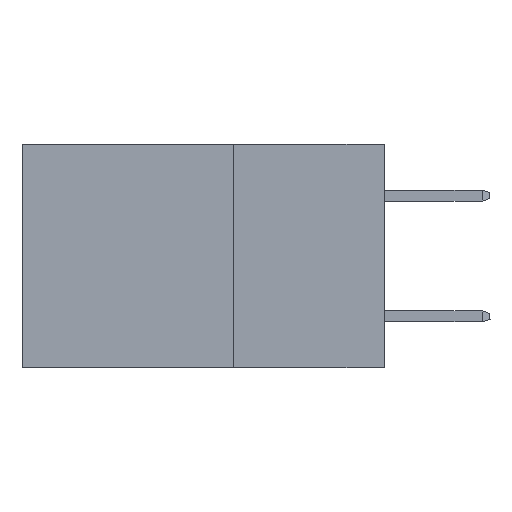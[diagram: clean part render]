
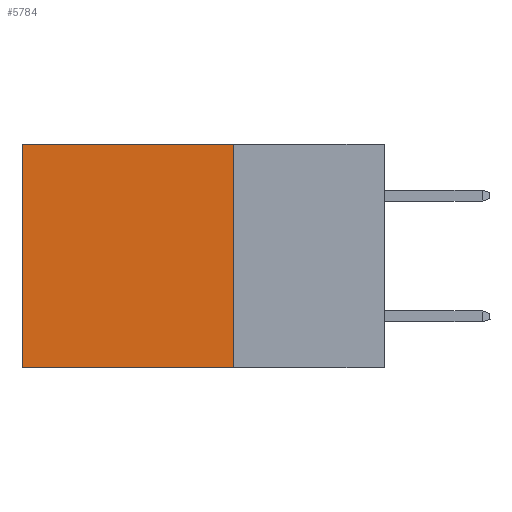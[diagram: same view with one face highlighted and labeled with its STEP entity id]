
A CAD part, left-side view. The second image highlights one B-rep face of the part: STEP entity #5784.
In plain terms, the highlighted planar face has unit normal (-1, 0, 0).
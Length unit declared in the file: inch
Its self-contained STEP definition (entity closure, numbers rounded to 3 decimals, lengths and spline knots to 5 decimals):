
#295 = PLANE ( 'NONE',  #4441 ) ;
#1437 = ORIENTED_EDGE ( 'NONE', *, *, #13617, .T. ) ;
#2033 = CARTESIAN_POINT ( 'NONE',  ( 0.2615, 0.25, -0.37 ) ) ;
#2458 = CARTESIAN_POINT ( 'NONE',  ( 0.2615, 0.25, 0. ) ) ;
#2679 = DIRECTION ( 'NONE',  ( 0., 0., -1. ) ) ;
#3398 = DIRECTION ( 'NONE',  ( 0., 1., 0. ) ) ;
#3536 = VECTOR ( 'NONE', #3398, 39.37008 ) ;
#3764 = DIRECTION ( 'NONE',  ( 1., 0., 0. ) ) ;
#4081 = LINE ( 'NONE', #8457, #3536 ) ;
#4148 = VERTEX_POINT ( 'NONE', #19362 ) ;
#4441 = AXIS2_PLACEMENT_3D ( 'NONE', #2033, #3764, #15387 ) ;
#5784 = ADVANCED_FACE ( 'NONE', ( #16815 ), #295, .F. ) ;
#7054 = EDGE_CURVE ( 'NONE', #9279, #13821, #4081, .T. ) ;
#7188 = VERTEX_POINT ( 'NONE', #13711 ) ;
#7354 = CARTESIAN_POINT ( 'NONE',  ( 0.2615, 0.25, -0.37 ) ) ;
#7905 = ORIENTED_EDGE ( 'NONE', *, *, #19389, .F. ) ;
#8277 = LINE ( 'NONE', #7354, #12148 ) ;
#8408 = LINE ( 'NONE', #19126, #16586 ) ;
#8457 = CARTESIAN_POINT ( 'NONE',  ( 0.2615, 0.25, 0. ) ) ;
#8946 = EDGE_LOOP ( 'NONE', ( #1437, #19120, #7905, #12744 ) ) ;
#9279 = VERTEX_POINT ( 'NONE', #2458 ) ;
#11519 = CARTESIAN_POINT ( 'NONE',  ( 0.2615, 0.6, 0. ) ) ;
#12148 = VECTOR ( 'NONE', #20444, 39.37008 ) ;
#12259 = LINE ( 'NONE', #17687, #20390 ) ;
#12744 = ORIENTED_EDGE ( 'NONE', *, *, #7054, .T. ) ;
#13617 = EDGE_CURVE ( 'NONE', #13821, #7188, #8408, .T. ) ;
#13711 = CARTESIAN_POINT ( 'NONE',  ( 0.2615, 0.6, -0.37 ) ) ;
#13821 = VERTEX_POINT ( 'NONE', #11519 ) ;
#15387 = DIRECTION ( 'NONE',  ( 0., 0., -1. ) ) ;
#16586 = VECTOR ( 'NONE', #2679, 39.37008 ) ;
#16815 = FACE_OUTER_BOUND ( 'NONE', #8946, .T. ) ;
#17191 = EDGE_CURVE ( 'NONE', #4148, #7188, #12259, .T. ) ;
#17687 = CARTESIAN_POINT ( 'NONE',  ( 0.2615, 0.25, -0.37 ) ) ;
#19120 = ORIENTED_EDGE ( 'NONE', *, *, #17191, .F. ) ;
#19126 = CARTESIAN_POINT ( 'NONE',  ( 0.2615, 0.6, -0.37 ) ) ;
#19335 = DIRECTION ( 'NONE',  ( 0., 1., 0. ) ) ;
#19362 = CARTESIAN_POINT ( 'NONE',  ( 0.2615, 0.25, -0.37 ) ) ;
#19389 = EDGE_CURVE ( 'NONE', #9279, #4148, #8277, .T. ) ;
#20390 = VECTOR ( 'NONE', #19335, 39.37008 ) ;
#20444 = DIRECTION ( 'NONE',  ( 0., 0., -1. ) ) ;
